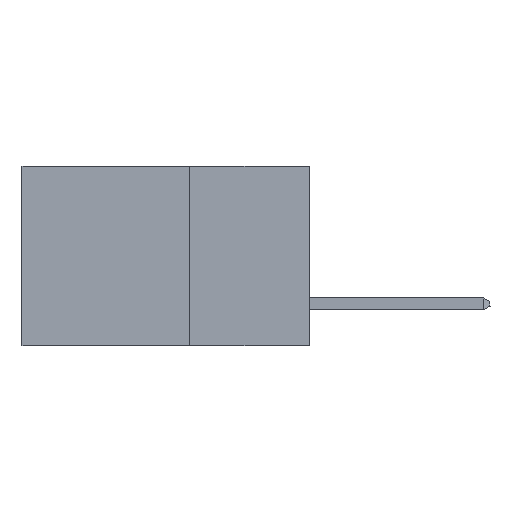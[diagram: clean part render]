
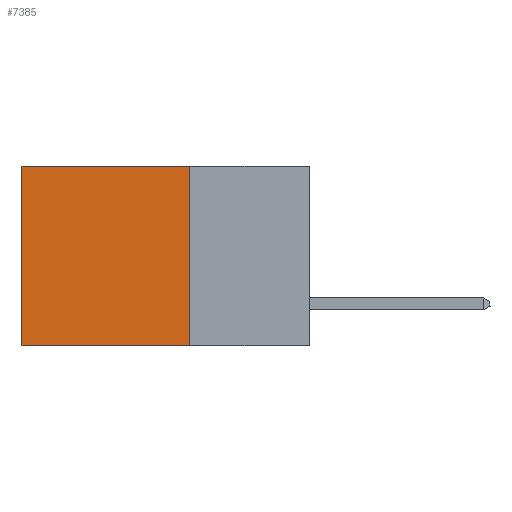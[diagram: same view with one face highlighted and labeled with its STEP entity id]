
A CAD part, left-side view. The second image highlights one B-rep face of the part: STEP entity #7385.
In plain terms, the highlighted planar face has unit normal (-1, 0, 0).
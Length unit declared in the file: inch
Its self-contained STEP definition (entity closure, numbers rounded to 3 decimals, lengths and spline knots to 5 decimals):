
#116 = CARTESIAN_POINT ( 'NONE',  ( 0.2875, 0.25, -0.375 ) ) ;
#1713 = ORIENTED_EDGE ( 'NONE', *, *, #18832, .F. ) ;
#1808 = DIRECTION ( 'NONE',  ( 0., 0., -1. ) ) ;
#2357 = VECTOR ( 'NONE', #10569, 39.37008 ) ;
#2619 = CARTESIAN_POINT ( 'NONE',  ( 0.2875, 0.25, 0. ) ) ;
#2844 = EDGE_CURVE ( 'NONE', #5907, #11735, #5330, .T. ) ;
#2976 = LINE ( 'NONE', #116, #12673 ) ;
#3042 = CARTESIAN_POINT ( 'NONE',  ( 0.2875, 0.25, 0. ) ) ;
#3322 = PLANE ( 'NONE',  #16083 ) ;
#3346 = CARTESIAN_POINT ( 'NONE',  ( 0.2875, 0.6, 0. ) ) ;
#3969 = ORIENTED_EDGE ( 'NONE', *, *, #11128, .F. ) ;
#4129 = VECTOR ( 'NONE', #16263, 39.37008 ) ;
#4479 = VERTEX_POINT ( 'NONE', #2619 ) ;
#5330 = LINE ( 'NONE', #13109, #11784 ) ;
#5619 = DIRECTION ( 'NONE',  ( 0., 0., -1. ) ) ;
#5907 = VERTEX_POINT ( 'NONE', #3346 ) ;
#7000 = DIRECTION ( 'NONE',  ( 0., 0., -1. ) ) ;
#7385 = ADVANCED_FACE ( 'NONE', ( #15125 ), #3322, .F. ) ;
#7683 = CARTESIAN_POINT ( 'NONE',  ( 0.2875, 0.25, -0.375 ) ) ;
#8366 = DIRECTION ( 'NONE',  ( 1., 0., 0. ) ) ;
#10569 = DIRECTION ( 'NONE',  ( 0., 1., 0. ) ) ;
#10798 = LINE ( 'NONE', #3042, #4129 ) ;
#11029 = CARTESIAN_POINT ( 'NONE',  ( 0.2875, 0.6, -0.375 ) ) ;
#11128 = EDGE_CURVE ( 'NONE', #4479, #13778, #2976, .T. ) ;
#11621 = ORIENTED_EDGE ( 'NONE', *, *, #15287, .T. ) ;
#11735 = VERTEX_POINT ( 'NONE', #11029 ) ;
#11784 = VECTOR ( 'NONE', #5619, 39.37008 ) ;
#12673 = VECTOR ( 'NONE', #1808, 39.37008 ) ;
#13109 = CARTESIAN_POINT ( 'NONE',  ( 0.2875, 0.6, -0.375 ) ) ;
#13651 = CARTESIAN_POINT ( 'NONE',  ( 0.2875, 0.25, -0.375 ) ) ;
#13778 = VERTEX_POINT ( 'NONE', #18294 ) ;
#15064 = LINE ( 'NONE', #7683, #2357 ) ;
#15125 = FACE_OUTER_BOUND ( 'NONE', #18091, .T. ) ;
#15287 = EDGE_CURVE ( 'NONE', #4479, #5907, #10798, .T. ) ;
#16083 = AXIS2_PLACEMENT_3D ( 'NONE', #13651, #8366, #7000 ) ;
#16263 = DIRECTION ( 'NONE',  ( 0., 1., 0. ) ) ;
#17197 = ORIENTED_EDGE ( 'NONE', *, *, #2844, .T. ) ;
#18091 = EDGE_LOOP ( 'NONE', ( #17197, #1713, #3969, #11621 ) ) ;
#18294 = CARTESIAN_POINT ( 'NONE',  ( 0.2875, 0.25, -0.375 ) ) ;
#18832 = EDGE_CURVE ( 'NONE', #13778, #11735, #15064, .T. ) ;
